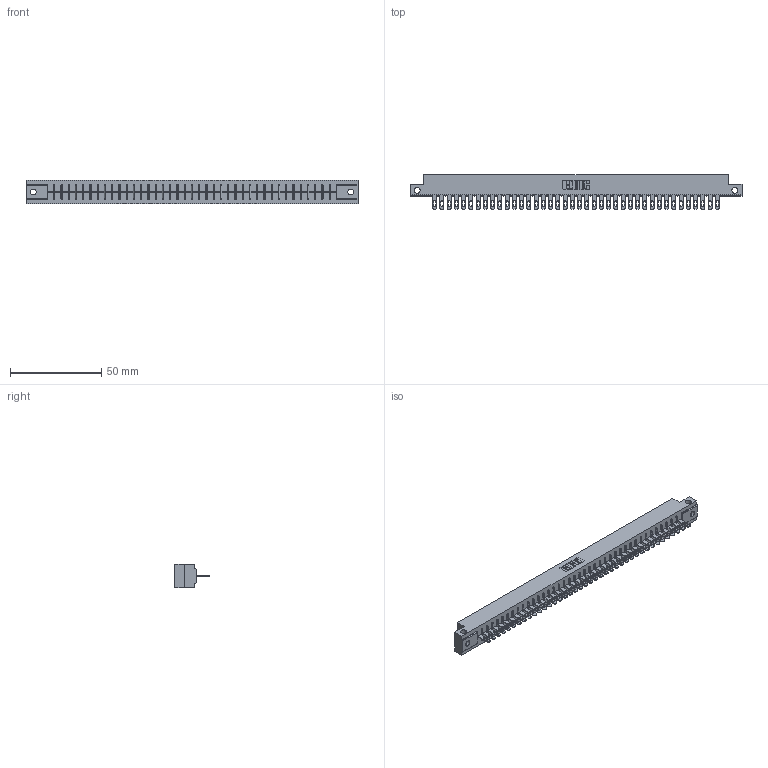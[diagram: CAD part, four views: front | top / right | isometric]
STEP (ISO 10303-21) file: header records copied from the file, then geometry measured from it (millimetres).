
FILE_DESCRIPTION (( 'STEP AP203' ), '1' );
FILE_NAME ('316-040-500-112.STEP', '2020-09-20T21:35:52', ( '' ), ( '' ), 'SwSTEP 2.0', 'SolidWorks 2020', '' );
FILE_SCHEMA (( 'CONFIG_CONTROL_DESIGN' ));
Length unit declared in the file: inch
Products named in the file (3): 316-040-500-112; 306-290-001_100; 306 Part_.128 Dia
Assembly tree (41 placements, depth 2):
  316-040-500-112
    306 Part_.128 Dia
    306-290-001_100  x40
Bounding box: 181.51 x 18.87 x 12.7 mm (x, y, z)
Volume: 19989.2 mm3; surface area: 21222.2 mm2
Topology: 41 solids, 41 shells, 3168 faces, 8952 edges, 5748 vertices
Faces by surface type: plane 2068, cylinder 940, sphere 160
Entity records: 38131 total; most frequent: CARTESIAN_POINT 6451, ORIENTED_EDGE 6352, DIRECTION 6300, EDGE_CURVE 3176, LINE 2466, VECTOR 2466, VERTEX_POINT 2004, AXIS2_PLACEMENT_3D 1917
